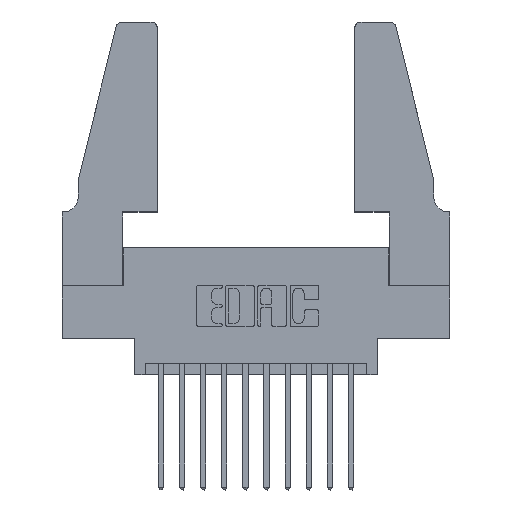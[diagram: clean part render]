
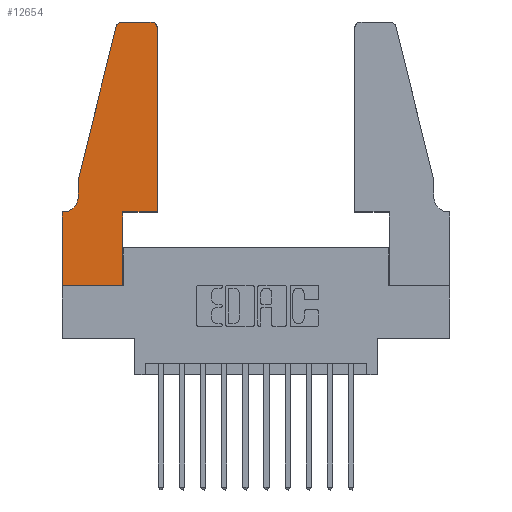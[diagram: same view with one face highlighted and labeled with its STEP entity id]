
A CAD part, top view. The second image highlights one B-rep face of the part: STEP entity #12654.
In plain terms, the highlighted planar face has unit normal (0, 0, 1).
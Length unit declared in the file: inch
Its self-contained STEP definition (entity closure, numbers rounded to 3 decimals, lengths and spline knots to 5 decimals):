
#251 = CARTESIAN_POINT ( 'NONE',  ( 0.2865, 0.35, 0.37 ) ) ;
#253 = DIRECTION ( 'NONE',  ( 1., 0., 0. ) ) ;
#495 = ORIENTED_EDGE ( 'NONE', *, *, #11853, .T. ) ;
#755 = DIRECTION ( 'NONE',  ( 0., 0., 1. ) ) ;
#950 = EDGE_CURVE ( 'NONE', #11050, #13506, #4484, .T. ) ;
#1026 = CARTESIAN_POINT ( 'NONE',  ( 0., 0.35, 0.37 ) ) ;
#1135 = VERTEX_POINT ( 'NONE', #2792 ) ;
#1205 = VECTOR ( 'NONE', #4157, 39.37008 ) ;
#1287 = LINE ( 'NONE', #11306, #12814 ) ;
#1553 = CARTESIAN_POINT ( 'NONE',  ( 0.0055, 0.35, 0.37 ) ) ;
#1568 = CARTESIAN_POINT ( 'NONE',  ( 0., 0., 0.37 ) ) ;
#1575 = ORIENTED_EDGE ( 'NONE', *, *, #10088, .T. ) ;
#1712 = ORIENTED_EDGE ( 'NONE', *, *, #9849, .T. ) ;
#1854 = VERTEX_POINT ( 'NONE', #251 ) ;
#2048 = CARTESIAN_POINT ( 'NONE',  ( 0.2605, 1.25, 0.37 ) ) ;
#2219 = DIRECTION ( 'NONE',  ( 0., 0., 1. ) ) ;
#2230 = CARTESIAN_POINT ( 'NONE',  ( 0.4505, 0.35, 0.37 ) ) ;
#2342 = VECTOR ( 'NONE', #3281, 39.37008 ) ;
#2566 = LINE ( 'NONE', #3033, #11831 ) ;
#2792 = CARTESIAN_POINT ( 'NONE',  ( 0.4205, 1.25, 0.37 ) ) ;
#2821 = DIRECTION ( 'NONE',  ( 0., 0., 1. ) ) ;
#2851 = CARTESIAN_POINT ( 'NONE',  ( 0., 0., 0.37 ) ) ;
#2889 = CARTESIAN_POINT ( 'NONE',  ( 0.0755, 0.35, 0.37 ) ) ;
#3033 = CARTESIAN_POINT ( 'NONE',  ( 0.2865, 0.35, 0.37 ) ) ;
#3085 = EDGE_CURVE ( 'NONE', #7989, #1135, #10071, .T. ) ;
#3135 = EDGE_CURVE ( 'NONE', #13890, #7989, #12531, .T. ) ;
#3281 = DIRECTION ( 'NONE',  ( -1., 0., 0. ) ) ;
#3392 = DIRECTION ( 'NONE',  ( -0.239, -0.971, 0. ) ) ;
#3819 = AXIS2_PLACEMENT_3D ( 'NONE', #12054, #5638, #13093 ) ;
#3878 = VERTEX_POINT ( 'NONE', #2851 ) ;
#4050 = CARTESIAN_POINT ( 'NONE',  ( 0.0755, 0.5, 0.37 ) ) ;
#4157 = DIRECTION ( 'NONE',  ( -1., 0., 0. ) ) ;
#4484 = LINE ( 'NONE', #2889, #1205 ) ;
#4515 = CARTESIAN_POINT ( 'NONE',  ( 0.0755, 0.42, 0.37 ) ) ;
#4739 = CIRCLE ( 'NONE', #3819, 0.07 ) ;
#4983 = VECTOR ( 'NONE', #11789, 39.37008 ) ;
#5074 = VECTOR ( 'NONE', #253, 39.37008 ) ;
#5201 = ORIENTED_EDGE ( 'NONE', *, *, #3085, .T. ) ;
#5282 = EDGE_CURVE ( 'NONE', #7533, #1854, #2566, .T. ) ;
#5354 = EDGE_CURVE ( 'NONE', #14396, #11050, #4739, .T. ) ;
#5534 = LINE ( 'NONE', #8851, #13688 ) ;
#5565 = AXIS2_PLACEMENT_3D ( 'NONE', #1026, #2219, #10160 ) ;
#5638 = DIRECTION ( 'NONE',  ( 0., 0., -1. ) ) ;
#5823 = ORIENTED_EDGE ( 'NONE', *, *, #13550, .T. ) ;
#6212 = ORIENTED_EDGE ( 'NONE', *, *, #3135, .T. ) ;
#6301 = LINE ( 'NONE', #11141, #8841 ) ;
#6633 = AXIS2_PLACEMENT_3D ( 'NONE', #9607, #2821, #10667 ) ;
#6952 = AXIS2_PLACEMENT_3D ( 'NONE', #7814, #755, #8869 ) ;
#7533 = VERTEX_POINT ( 'NONE', #9110 ) ;
#7589 = EDGE_CURVE ( 'NONE', #9080, #14396, #1287, .T. ) ;
#7814 = CARTESIAN_POINT ( 'NONE',  ( 0.284, 1.22, 0.37 ) ) ;
#7989 = VERTEX_POINT ( 'NONE', #14031 ) ;
#8055 = PLANE ( 'NONE',  #5565 ) ;
#8314 = CIRCLE ( 'NONE', #6952, 0.03 ) ;
#8841 = VECTOR ( 'NONE', #3392, 39.37008 ) ;
#8851 = CARTESIAN_POINT ( 'NONE',  ( 0.4505, 0.35, 0.37 ) ) ;
#8869 = DIRECTION ( 'NONE',  ( 1., 0., 0. ) ) ;
#8999 = LINE ( 'NONE', #9631, #11805 ) ;
#9080 = VERTEX_POINT ( 'NONE', #4050 ) ;
#9110 = CARTESIAN_POINT ( 'NONE',  ( 0.2865, 0., 0.37 ) ) ;
#9607 = CARTESIAN_POINT ( 'NONE',  ( 0.4205, 1.22, 0.37 ) ) ;
#9631 = CARTESIAN_POINT ( 'NONE',  ( 0., 0., 0.37 ) ) ;
#9849 = EDGE_CURVE ( 'NONE', #13506, #3878, #8999, .T. ) ;
#10023 = ORIENTED_EDGE ( 'NONE', *, *, #950, .T. ) ;
#10071 = CIRCLE ( 'NONE', #6633, 0.03 ) ;
#10088 = EDGE_CURVE ( 'NONE', #1135, #12718, #11287, .T. ) ;
#10158 = ORIENTED_EDGE ( 'NONE', *, *, #11223, .T. ) ;
#10160 = DIRECTION ( 'NONE',  ( 1., 0., 0. ) ) ;
#10248 = CARTESIAN_POINT ( 'NONE',  ( 0.284, 1.25, 0.37 ) ) ;
#10408 = ORIENTED_EDGE ( 'NONE', *, *, #7589, .T. ) ;
#10667 = DIRECTION ( 'NONE',  ( 1., 0., 0. ) ) ;
#10713 = CARTESIAN_POINT ( 'NONE',  ( 0.4505, 0.35, 0.37 ) ) ;
#10846 = DIRECTION ( 'NONE',  ( 0., 1., 0. ) ) ;
#11050 = VERTEX_POINT ( 'NONE', #1553 ) ;
#11063 = CARTESIAN_POINT ( 'NONE',  ( 0.25487, 1.22718, 0.37 ) ) ;
#11114 = EDGE_LOOP ( 'NONE', ( #1575, #10158, #11646, #10408, #14096, #10023, #1712, #5823, #11380, #495, #6212, #5201 ) ) ;
#11130 = LINE ( 'NONE', #1568, #5074 ) ;
#11141 = CARTESIAN_POINT ( 'NONE',  ( 0.0755, 0.5, 0.37 ) ) ;
#11162 = FACE_OUTER_BOUND ( 'NONE', #11114, .T. ) ;
#11223 = EDGE_CURVE ( 'NONE', #12718, #12597, #8314, .T. ) ;
#11287 = LINE ( 'NONE', #2048, #2342 ) ;
#11306 = CARTESIAN_POINT ( 'NONE',  ( 0.0755, 0.5, 0.37 ) ) ;
#11380 = ORIENTED_EDGE ( 'NONE', *, *, #5282, .T. ) ;
#11611 = CARTESIAN_POINT ( 'NONE',  ( 0., 0.35, 0.37 ) ) ;
#11646 = ORIENTED_EDGE ( 'NONE', *, *, #13251, .T. ) ;
#11765 = DIRECTION ( 'NONE',  ( 0., -1., 0. ) ) ;
#11789 = DIRECTION ( 'NONE',  ( 0., 1., 0. ) ) ;
#11805 = VECTOR ( 'NONE', #11765, 39.37008 ) ;
#11831 = VECTOR ( 'NONE', #10846, 39.37008 ) ;
#11853 = EDGE_CURVE ( 'NONE', #1854, #13890, #5534, .T. ) ;
#12025 = DIRECTION ( 'NONE',  ( 1., 0., 0. ) ) ;
#12054 = CARTESIAN_POINT ( 'NONE',  ( 0.0055, 0.42, 0.37 ) ) ;
#12531 = LINE ( 'NONE', #10713, #4983 ) ;
#12597 = VERTEX_POINT ( 'NONE', #11063 ) ;
#12654 = ADVANCED_FACE ( 'NONE', ( #11162 ), #8055, .T. ) ;
#12718 = VERTEX_POINT ( 'NONE', #10248 ) ;
#12814 = VECTOR ( 'NONE', #13412, 39.37008 ) ;
#13093 = DIRECTION ( 'NONE',  ( -1., 0., 0. ) ) ;
#13251 = EDGE_CURVE ( 'NONE', #12597, #9080, #6301, .T. ) ;
#13412 = DIRECTION ( 'NONE',  ( 0., -1., 0. ) ) ;
#13506 = VERTEX_POINT ( 'NONE', #11611 ) ;
#13550 = EDGE_CURVE ( 'NONE', #3878, #7533, #11130, .T. ) ;
#13688 = VECTOR ( 'NONE', #12025, 39.37008 ) ;
#13890 = VERTEX_POINT ( 'NONE', #2230 ) ;
#14031 = CARTESIAN_POINT ( 'NONE',  ( 0.4505, 1.22, 0.37 ) ) ;
#14096 = ORIENTED_EDGE ( 'NONE', *, *, #5354, .T. ) ;
#14396 = VERTEX_POINT ( 'NONE', #4515 ) ;
